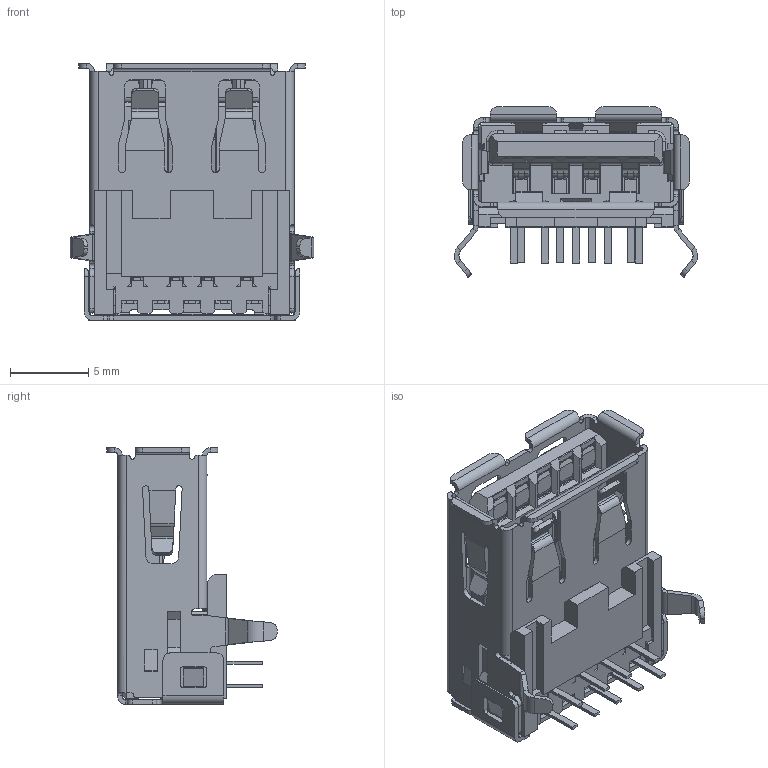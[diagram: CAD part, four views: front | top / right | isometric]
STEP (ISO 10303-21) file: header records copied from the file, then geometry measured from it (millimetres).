
FILE_DESCRIPTION (( 'STEP AP214' ), '1' );
FILE_NAME ('690B109-123-012.STEP', '2021-01-14T17:24:16', ( '' ), ( '' ), 'SwSTEP 2.0', 'SolidWorks 2020', '' );
FILE_SCHEMA (( 'AUTOMOTIVE_DESIGN' ));
Length unit declared in the file: millimetre
Products named in the file (4): Contacts 690B109-X23-0X2; Insulator 690B109-X23-0X2; 690B109-123-012; Shell 690B109-X23-0X2
Assembly tree (3 placements, depth 2):
  690B109-123-012
    Insulator 690B109-X23-0X2
    Contacts 690B109-X23-0X2
    Shell 690B109-X23-0X2
Bounding box: 15.6 x 10.92 x 16.45 mm (x, y, z)
Volume: 676.9 mm3; surface area: 3042.5 mm2
Topology: 11 solids, 11 shells, 2295 faces, 6701 edges, 4359 vertices
Faces by surface type: plane 1564, cylinder 593, bspline 130, torus 8
Entity records: 78521 total; most frequent: CARTESIAN_POINT 17810, ORIENTED_EDGE 13402, DIRECTION 11761, EDGE_CURVE 6701, LINE 5221, VECTOR 5221, VERTEX_POINT 4359, AXIS2_PLACEMENT_3D 3270
